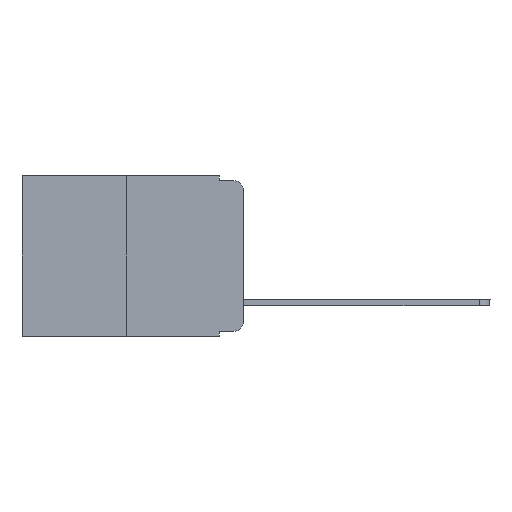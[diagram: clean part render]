
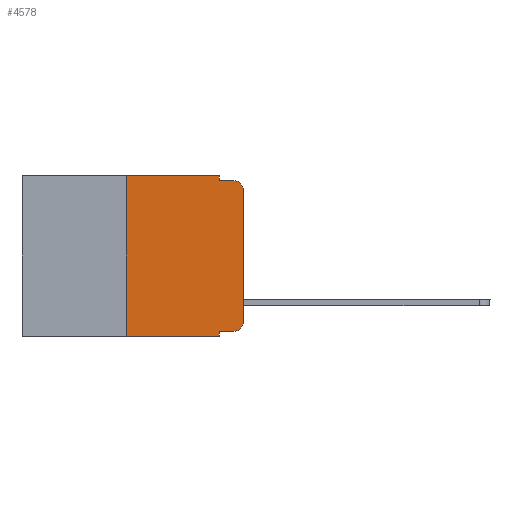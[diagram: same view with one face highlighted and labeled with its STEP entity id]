
A CAD part, left-side view. The second image highlights one B-rep face of the part: STEP entity #4578.
In plain terms, the highlighted planar face has unit normal (-1, 0, 0).
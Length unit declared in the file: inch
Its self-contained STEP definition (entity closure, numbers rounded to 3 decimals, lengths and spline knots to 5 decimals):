
#188 = VERTEX_POINT ( 'NONE', #8233 ) ;
#316 = ORIENTED_EDGE ( 'NONE', *, *, #11756, .F. ) ;
#493 = EDGE_LOOP ( 'NONE', ( #13388, #17780, #316, #13452, #5846, #6364, #13473, #7531, #1302, #18335 ) ) ;
#676 = EDGE_CURVE ( 'NONE', #15989, #13024, #6564, .T. ) ;
#1200 = CARTESIAN_POINT ( 'NONE',  ( 0., 0.25, -0.343 ) ) ;
#1291 = EDGE_CURVE ( 'NONE', #19134, #188, #12624, .T. ) ;
#1302 = ORIENTED_EDGE ( 'NONE', *, *, #15669, .T. ) ;
#1403 = CARTESIAN_POINT ( 'NONE',  ( 0., 0.051, 0. ) ) ;
#1426 = CARTESIAN_POINT ( 'NONE',  ( 0., 0.051, 0. ) ) ;
#2381 = CARTESIAN_POINT ( 'NONE',  ( 0., 0.051, 0. ) ) ;
#2386 = PLANE ( 'NONE',  #9052 ) ;
#2568 = VECTOR ( 'NONE', #10635, 39.37008 ) ;
#2822 = CARTESIAN_POINT ( 'NONE',  ( 0., 0.02, -0.01 ) ) ;
#2887 = CARTESIAN_POINT ( 'NONE',  ( 0., 0.051, -0.01 ) ) ;
#3123 = VECTOR ( 'NONE', #4002, 39.37008 ) ;
#3161 = EDGE_CURVE ( 'NONE', #9605, #15989, #19881, .T. ) ;
#3559 = VERTEX_POINT ( 'NONE', #14163 ) ;
#3657 = CARTESIAN_POINT ( 'NONE',  ( 0., 0., -0.03 ) ) ;
#3899 = EDGE_CURVE ( 'NONE', #13024, #10123, #13336, .T. ) ;
#4002 = DIRECTION ( 'NONE',  ( 0., -1., 0. ) ) ;
#4578 = ADVANCED_FACE ( 'NONE', ( #5474 ), #2386, .F. ) ;
#5240 = CARTESIAN_POINT ( 'NONE',  ( 0., 0.473, 0. ) ) ;
#5431 = CARTESIAN_POINT ( 'NONE',  ( 0., 0., -0.313 ) ) ;
#5474 = FACE_OUTER_BOUND ( 'NONE', #493, .T. ) ;
#5591 = VECTOR ( 'NONE', #8210, 39.37008 ) ;
#5846 = ORIENTED_EDGE ( 'NONE', *, *, #17280, .F. ) ;
#5882 = DIRECTION ( 'NONE',  ( 0., 0., -1. ) ) ;
#6133 = LINE ( 'NONE', #12487, #2568 ) ;
#6364 = ORIENTED_EDGE ( 'NONE', *, *, #6767, .F. ) ;
#6564 = LINE ( 'NONE', #8304, #5591 ) ;
#6767 = EDGE_CURVE ( 'NONE', #19134, #18046, #6133, .T. ) ;
#6886 = LINE ( 'NONE', #5240, #3123 ) ;
#7531 = ORIENTED_EDGE ( 'NONE', *, *, #11819, .F. ) ;
#7649 = VECTOR ( 'NONE', #12209, 39.37008 ) ;
#7687 = VECTOR ( 'NONE', #17260, 39.37008 ) ;
#7930 = VECTOR ( 'NONE', #18198, 39.37008 ) ;
#8210 = DIRECTION ( 'NONE',  ( 0., 0., 1. ) ) ;
#8233 = CARTESIAN_POINT ( 'NONE',  ( 0., 0.051, -0.343 ) ) ;
#8258 = DIRECTION ( 'NONE',  ( 0., 0., -1. ) ) ;
#8304 = CARTESIAN_POINT ( 'NONE',  ( 0., 0., 0. ) ) ;
#8355 = CARTESIAN_POINT ( 'NONE',  ( 0., 0.02, -0.313 ) ) ;
#8650 = DIRECTION ( 'NONE',  ( 1., 0., 0. ) ) ;
#8933 = CARTESIAN_POINT ( 'NONE',  ( 0., 0.051, -0.333 ) ) ;
#9052 = AXIS2_PLACEMENT_3D ( 'NONE', #13170, #8650, #19648 ) ;
#9605 = VERTEX_POINT ( 'NONE', #11502 ) ;
#10123 = VERTEX_POINT ( 'NONE', #2822 ) ;
#10178 = LINE ( 'NONE', #2381, #14470 ) ;
#10635 = DIRECTION ( 'NONE',  ( 0., 0., 1. ) ) ;
#10916 = CARTESIAN_POINT ( 'NONE',  ( 0., 0.25, 0. ) ) ;
#10977 = CARTESIAN_POINT ( 'NONE',  ( 0., 0.473, -0.343 ) ) ;
#11006 = AXIS2_PLACEMENT_3D ( 'NONE', #8355, #19341, #8258 ) ;
#11502 = CARTESIAN_POINT ( 'NONE',  ( 0., 0.02, -0.333 ) ) ;
#11756 = EDGE_CURVE ( 'NONE', #11899, #10123, #14810, .T. ) ;
#11819 = EDGE_CURVE ( 'NONE', #3559, #188, #10178, .T. ) ;
#11899 = VERTEX_POINT ( 'NONE', #2887 ) ;
#11915 = CARTESIAN_POINT ( 'NONE',  ( 0., 0.051, -0.01 ) ) ;
#12209 = DIRECTION ( 'NONE',  ( 0., -1., 0. ) ) ;
#12398 = DIRECTION ( 'NONE',  ( -1., 0., 0. ) ) ;
#12487 = CARTESIAN_POINT ( 'NONE',  ( 0., 0.25, 0. ) ) ;
#12624 = LINE ( 'NONE', #10977, #7687 ) ;
#13024 = VERTEX_POINT ( 'NONE', #3657 ) ;
#13170 = CARTESIAN_POINT ( 'NONE',  ( 0., 0.473, 0. ) ) ;
#13336 = CIRCLE ( 'NONE', #15971, 0.02 ) ;
#13388 = ORIENTED_EDGE ( 'NONE', *, *, #676, .T. ) ;
#13452 = ORIENTED_EDGE ( 'NONE', *, *, #15231, .F. ) ;
#13473 = ORIENTED_EDGE ( 'NONE', *, *, #1291, .T. ) ;
#13524 = VECTOR ( 'NONE', #5882, 39.37008 ) ;
#14163 = CARTESIAN_POINT ( 'NONE',  ( 0., 0.051, -0.333 ) ) ;
#14352 = LINE ( 'NONE', #1426, #13524 ) ;
#14470 = VECTOR ( 'NONE', #16355, 39.37008 ) ;
#14810 = LINE ( 'NONE', #11915, #7930 ) ;
#15231 = EDGE_CURVE ( 'NONE', #19154, #11899, #14352, .T. ) ;
#15398 = LINE ( 'NONE', #8933, #7649 ) ;
#15669 = EDGE_CURVE ( 'NONE', #3559, #9605, #15398, .T. ) ;
#15971 = AXIS2_PLACEMENT_3D ( 'NONE', #20213, #12398, #18678 ) ;
#15989 = VERTEX_POINT ( 'NONE', #5431 ) ;
#16355 = DIRECTION ( 'NONE',  ( 0., 0., -1. ) ) ;
#17260 = DIRECTION ( 'NONE',  ( 0., -1., 0. ) ) ;
#17280 = EDGE_CURVE ( 'NONE', #18046, #19154, #6886, .T. ) ;
#17780 = ORIENTED_EDGE ( 'NONE', *, *, #3899, .T. ) ;
#18046 = VERTEX_POINT ( 'NONE', #10916 ) ;
#18198 = DIRECTION ( 'NONE',  ( 0., -1., 0. ) ) ;
#18335 = ORIENTED_EDGE ( 'NONE', *, *, #3161, .T. ) ;
#18678 = DIRECTION ( 'NONE',  ( 0., 0., -1. ) ) ;
#19134 = VERTEX_POINT ( 'NONE', #1200 ) ;
#19154 = VERTEX_POINT ( 'NONE', #1403 ) ;
#19341 = DIRECTION ( 'NONE',  ( -1., 0., 0. ) ) ;
#19648 = DIRECTION ( 'NONE',  ( 0., 0., -1. ) ) ;
#19881 = CIRCLE ( 'NONE', #11006, 0.02 ) ;
#20213 = CARTESIAN_POINT ( 'NONE',  ( 0., 0.02, -0.03 ) ) ;
